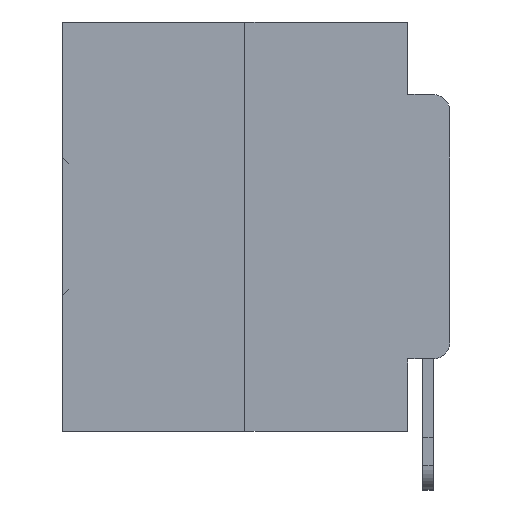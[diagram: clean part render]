
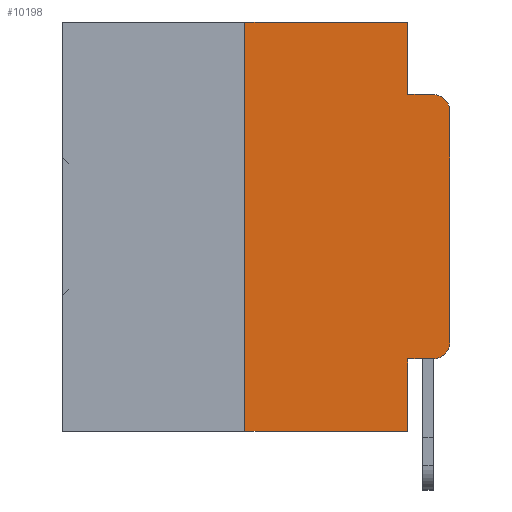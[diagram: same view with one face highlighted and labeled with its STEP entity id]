
A CAD part, left-side view. The second image highlights one B-rep face of the part: STEP entity #10198.
In plain terms, the highlighted planar face has unit normal (-1, 0, 0).
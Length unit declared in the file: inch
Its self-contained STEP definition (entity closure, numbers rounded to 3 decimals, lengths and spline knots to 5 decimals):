
#105 = AXIS2_PLACEMENT_3D ( 'NONE', #27000, #21679, #4930 ) ;
#376 = EDGE_CURVE ( 'NONE', #14263, #20236, #13131, .T. ) ;
#419 = VERTEX_POINT ( 'NONE', #5560 ) ;
#686 = CARTESIAN_POINT ( 'NONE',  ( 0., 0.051, -0.4115 ) ) ;
#1458 = VECTOR ( 'NONE', #26399, 39.37008 ) ;
#2391 = ORIENTED_EDGE ( 'NONE', *, *, #26569, .T. ) ;
#3198 = DIRECTION ( 'NONE',  ( -1., 0., 0. ) ) ;
#3299 = LINE ( 'NONE', #10804, #26359 ) ;
#3496 = ORIENTED_EDGE ( 'NONE', *, *, #24758, .T. ) ;
#3823 = DIRECTION ( 'NONE',  ( 0., 0., -1. ) ) ;
#4355 = CARTESIAN_POINT ( 'NONE',  ( 0., 0., 0. ) ) ;
#4477 = DIRECTION ( 'NONE',  ( 0., -1., 0. ) ) ;
#4629 = CARTESIAN_POINT ( 'NONE',  ( 0., 0.051, -0.0885 ) ) ;
#4709 = DIRECTION ( 'NONE',  ( 0., 0., -1. ) ) ;
#4930 = DIRECTION ( 'NONE',  ( 0., 0., -1. ) ) ;
#5522 = ORIENTED_EDGE ( 'NONE', *, *, #22994, .F. ) ;
#5560 = CARTESIAN_POINT ( 'NONE',  ( 0., 0.051, -0.0885 ) ) ;
#5885 = ORIENTED_EDGE ( 'NONE', *, *, #13702, .F. ) ;
#6713 = CARTESIAN_POINT ( 'NONE',  ( 0., 0.02, -0.0885 ) ) ;
#7044 = ORIENTED_EDGE ( 'NONE', *, *, #35520, .F. ) ;
#7887 = AXIS2_PLACEMENT_3D ( 'NONE', #29914, #13508, #32653 ) ;
#8538 = ORIENTED_EDGE ( 'NONE', *, *, #11839, .F. ) ;
#8549 = CIRCLE ( 'NONE', #28934, 0.02 ) ;
#8970 = FACE_OUTER_BOUND ( 'NONE', #35047, .T. ) ;
#9890 = DIRECTION ( 'NONE',  ( 0., -1., 0. ) ) ;
#9942 = EDGE_CURVE ( 'NONE', #14263, #29265, #31380, .T. ) ;
#10198 = ADVANCED_FACE ( 'NONE', ( #8970 ), #18907, .F. ) ;
#10217 = DIRECTION ( 'NONE',  ( 0., -1., 0. ) ) ;
#10329 = CARTESIAN_POINT ( 'NONE',  ( 0., 0.051, -0.5 ) ) ;
#10804 = CARTESIAN_POINT ( 'NONE',  ( 0., 0.473, -0.5 ) ) ;
#11376 = ORIENTED_EDGE ( 'NONE', *, *, #21389, .T. ) ;
#11839 = EDGE_CURVE ( 'NONE', #24537, #19159, #23804, .T. ) ;
#11974 = ORIENTED_EDGE ( 'NONE', *, *, #9942, .F. ) ;
#13044 = CARTESIAN_POINT ( 'NONE',  ( 0., 0.051, 0. ) ) ;
#13131 = LINE ( 'NONE', #686, #34083 ) ;
#13508 = DIRECTION ( 'NONE',  ( -1., 0., 0. ) ) ;
#13702 = EDGE_CURVE ( 'NONE', #23928, #419, #34664, .T. ) ;
#14071 = ORIENTED_EDGE ( 'NONE', *, *, #376, .T. ) ;
#14263 = VERTEX_POINT ( 'NONE', #19927 ) ;
#15041 = CARTESIAN_POINT ( 'NONE',  ( 0., 0.051, 0. ) ) ;
#15297 = CARTESIAN_POINT ( 'NONE',  ( 0., 0., -0.1085 ) ) ;
#15694 = DIRECTION ( 'NONE',  ( 0., 0., 1. ) ) ;
#15873 = LINE ( 'NONE', #23731, #22357 ) ;
#15902 = CARTESIAN_POINT ( 'NONE',  ( 0., 0.051, 0. ) ) ;
#16374 = ORIENTED_EDGE ( 'NONE', *, *, #34537, .T. ) ;
#17416 = CIRCLE ( 'NONE', #7887, 0.02 ) ;
#17471 = CARTESIAN_POINT ( 'NONE',  ( 0., 0., -0.3915 ) ) ;
#18907 = PLANE ( 'NONE',  #105 ) ;
#19159 = VERTEX_POINT ( 'NONE', #27316 ) ;
#19927 = CARTESIAN_POINT ( 'NONE',  ( 0., 0.051, -0.4115 ) ) ;
#20040 = CARTESIAN_POINT ( 'NONE',  ( 0., 0.02, -0.1085 ) ) ;
#20236 = VERTEX_POINT ( 'NONE', #25894 ) ;
#20880 = VERTEX_POINT ( 'NONE', #6713 ) ;
#21075 = LINE ( 'NONE', #4355, #27418 ) ;
#21389 = EDGE_CURVE ( 'NONE', #24537, #29265, #3299, .T. ) ;
#21679 = DIRECTION ( 'NONE',  ( 1., 0., 0. ) ) ;
#22067 = VECTOR ( 'NONE', #10217, 39.37008 ) ;
#22357 = VECTOR ( 'NONE', #9890, 39.37008 ) ;
#22782 = DIRECTION ( 'NONE',  ( 0., 0., -1. ) ) ;
#22994 = EDGE_CURVE ( 'NONE', #419, #20880, #30129, .T. ) ;
#23716 = CARTESIAN_POINT ( 'NONE',  ( 0., 0.25, 0. ) ) ;
#23731 = CARTESIAN_POINT ( 'NONE',  ( 0., 0.473, 0. ) ) ;
#23804 = LINE ( 'NONE', #23716, #1458 ) ;
#23928 = VERTEX_POINT ( 'NONE', #13044 ) ;
#24185 = VECTOR ( 'NONE', #3823, 39.37008 ) ;
#24537 = VERTEX_POINT ( 'NONE', #35338 ) ;
#24758 = EDGE_CURVE ( 'NONE', #33168, #20880, #8549, .T. ) ;
#25894 = CARTESIAN_POINT ( 'NONE',  ( 0., 0.02, -0.4115 ) ) ;
#26359 = VECTOR ( 'NONE', #30031, 39.37008 ) ;
#26399 = DIRECTION ( 'NONE',  ( 0., 0., 1. ) ) ;
#26569 = EDGE_CURVE ( 'NONE', #28987, #33168, #21075, .T. ) ;
#27000 = CARTESIAN_POINT ( 'NONE',  ( 0., 0.473, 0. ) ) ;
#27316 = CARTESIAN_POINT ( 'NONE',  ( 0., 0.25, 0. ) ) ;
#27418 = VECTOR ( 'NONE', #15694, 39.37008 ) ;
#27419 = VECTOR ( 'NONE', #4709, 39.37008 ) ;
#28934 = AXIS2_PLACEMENT_3D ( 'NONE', #20040, #3198, #22782 ) ;
#28987 = VERTEX_POINT ( 'NONE', #17471 ) ;
#29265 = VERTEX_POINT ( 'NONE', #10329 ) ;
#29914 = CARTESIAN_POINT ( 'NONE',  ( 0., 0.02, -0.3915 ) ) ;
#30031 = DIRECTION ( 'NONE',  ( 0., -1., 0. ) ) ;
#30129 = LINE ( 'NONE', #4629, #22067 ) ;
#31380 = LINE ( 'NONE', #15041, #24185 ) ;
#32653 = DIRECTION ( 'NONE',  ( 0., 0., -1. ) ) ;
#33168 = VERTEX_POINT ( 'NONE', #15297 ) ;
#34083 = VECTOR ( 'NONE', #4477, 39.37008 ) ;
#34537 = EDGE_CURVE ( 'NONE', #20236, #28987, #17416, .T. ) ;
#34664 = LINE ( 'NONE', #15902, #27419 ) ;
#35047 = EDGE_LOOP ( 'NONE', ( #2391, #3496, #5522, #5885, #7044, #8538, #11376, #11974, #14071, #16374 ) ) ;
#35338 = CARTESIAN_POINT ( 'NONE',  ( 0., 0.25, -0.5 ) ) ;
#35520 = EDGE_CURVE ( 'NONE', #19159, #23928, #15873, .T. ) ;
